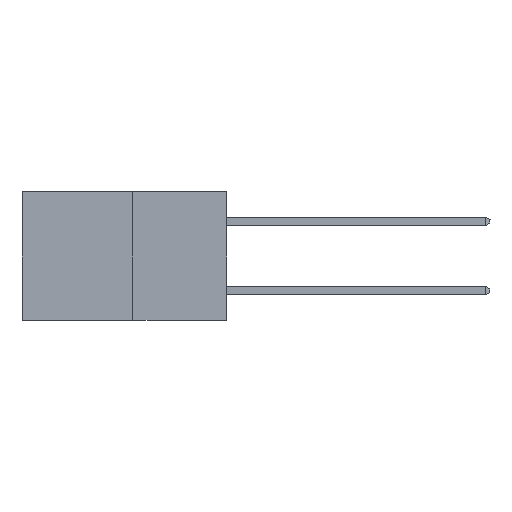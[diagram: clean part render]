
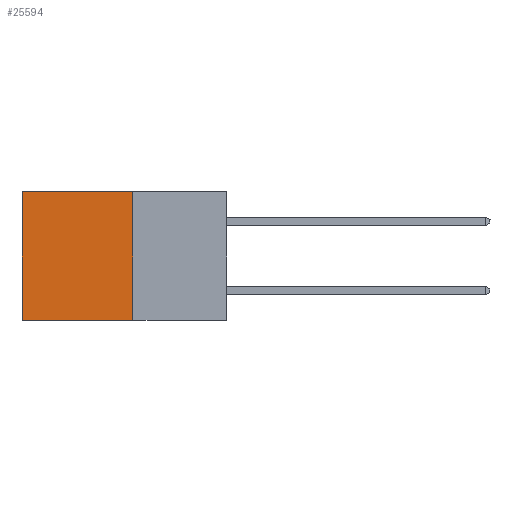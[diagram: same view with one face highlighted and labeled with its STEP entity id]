
A CAD part, left-side view. The second image highlights one B-rep face of the part: STEP entity #25594.
In plain terms, the highlighted planar face has unit normal (-1, 0, 0).
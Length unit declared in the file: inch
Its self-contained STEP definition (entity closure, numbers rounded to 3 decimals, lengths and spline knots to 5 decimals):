
#349 = VECTOR ( 'NONE', #24179, 39.37008 ) ;
#362 = EDGE_LOOP ( 'NONE', ( #29598, #16596, #34084, #12481 ) ) ;
#2680 = LINE ( 'NONE', #28192, #30081 ) ;
#3738 = CARTESIAN_POINT ( 'NONE',  ( 0.277, 0.59, -0.37 ) ) ;
#4089 = DIRECTION ( 'NONE',  ( 0., 1., 0. ) ) ;
#8276 = VERTEX_POINT ( 'NONE', #28508 ) ;
#8285 = CARTESIAN_POINT ( 'NONE',  ( 0.277, 0.27, -0.37 ) ) ;
#10663 = CARTESIAN_POINT ( 'NONE',  ( 0.277, 0.27, -0.37 ) ) ;
#10864 = VERTEX_POINT ( 'NONE', #3738 ) ;
#11669 = CARTESIAN_POINT ( 'NONE',  ( 0.277, 0.59, 0. ) ) ;
#11889 = VERTEX_POINT ( 'NONE', #20705 ) ;
#12481 = ORIENTED_EDGE ( 'NONE', *, *, #13074, .T. ) ;
#13074 = EDGE_CURVE ( 'NONE', #11889, #33313, #21058, .T. ) ;
#13365 = DIRECTION ( 'NONE',  ( 0., 0., -1. ) ) ;
#14634 = LINE ( 'NONE', #32028, #349 ) ;
#14840 = VECTOR ( 'NONE', #4089, 39.37008 ) ;
#15055 = DIRECTION ( 'NONE',  ( 0., 0., -1. ) ) ;
#16596 = ORIENTED_EDGE ( 'NONE', *, *, #26151, .F. ) ;
#20057 = CARTESIAN_POINT ( 'NONE',  ( 0.277, 0.27, 0. ) ) ;
#20705 = CARTESIAN_POINT ( 'NONE',  ( 0.277, 0.27, 0. ) ) ;
#21058 = LINE ( 'NONE', #20057, #14840 ) ;
#22959 = AXIS2_PLACEMENT_3D ( 'NONE', #10663, #29153, #13365 ) ;
#22990 = EDGE_CURVE ( 'NONE', #11889, #8276, #14634, .T. ) ;
#24179 = DIRECTION ( 'NONE',  ( 0., 0., -1. ) ) ;
#25594 = ADVANCED_FACE ( 'NONE', ( #30543 ), #26540, .F. ) ;
#26151 = EDGE_CURVE ( 'NONE', #8276, #10864, #31708, .T. ) ;
#26540 = PLANE ( 'NONE',  #22959 ) ;
#26853 = DIRECTION ( 'NONE',  ( 0., 1., 0. ) ) ;
#28192 = CARTESIAN_POINT ( 'NONE',  ( 0.277, 0.59, -0.37 ) ) ;
#28508 = CARTESIAN_POINT ( 'NONE',  ( 0.277, 0.27, -0.37 ) ) ;
#29153 = DIRECTION ( 'NONE',  ( 1., 0., 0. ) ) ;
#29598 = ORIENTED_EDGE ( 'NONE', *, *, #32065, .T. ) ;
#30081 = VECTOR ( 'NONE', #15055, 39.37008 ) ;
#30543 = FACE_OUTER_BOUND ( 'NONE', #362, .T. ) ;
#30911 = VECTOR ( 'NONE', #26853, 39.37008 ) ;
#31708 = LINE ( 'NONE', #8285, #30911 ) ;
#32028 = CARTESIAN_POINT ( 'NONE',  ( 0.277, 0.27, -0.37 ) ) ;
#32065 = EDGE_CURVE ( 'NONE', #33313, #10864, #2680, .T. ) ;
#33313 = VERTEX_POINT ( 'NONE', #11669 ) ;
#34084 = ORIENTED_EDGE ( 'NONE', *, *, #22990, .F. ) ;
